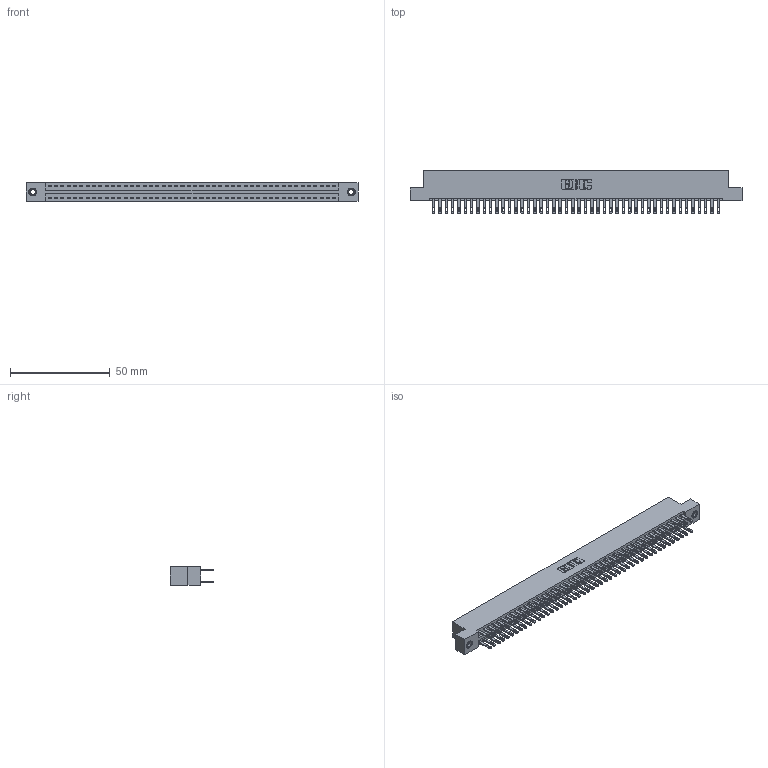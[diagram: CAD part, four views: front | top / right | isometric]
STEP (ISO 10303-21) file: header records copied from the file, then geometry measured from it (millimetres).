
FILE_DESCRIPTION (( 'STEP AP203' ), '1' );
FILE_NAME ('346-092-500-207.STEP', '2022-05-26T05:49:21', ( '' ), ( '' ), 'SwSTEP 2.0', 'SolidWorks 2020', '' );
FILE_SCHEMA (( 'CONFIG_CONTROL_DESIGN' ));
Length unit declared in the file: inch
Products named in the file (4): 346 Part_Flush Mounting Lugs - 0.156 Dia-TI; 346-092-500-207; 345-250-001_345-250-005-103; 345-292-001_345-293-100
Assembly tree (95 placements, depth 2):
  346-092-500-207
    346 Part_Flush Mounting Lugs - 0.156 Dia-TI
    345-292-001_345-293-100  x92
    345-250-001_345-250-005-103  x2
Bounding box: 166.62 x 21.84 x 9.4 mm (x, y, z)
Volume: 16546.6 mm3; surface area: 23804 mm2
Topology: 95 solids, 95 shells, 4598 faces, 13989 edges, 9318 vertices
Faces by surface type: plane 2776, cylinder 1806, cone 12, torus 4
Entity records: 30598 total; most frequent: CARTESIAN_POINT 5019, ORIENTED_EDGE 4946, DIRECTION 4503, EDGE_CURVE 2473, VECTOR 2133, LINE 2133, VERTEX_POINT 1644, AXIS2_PLACEMENT_3D 1185
